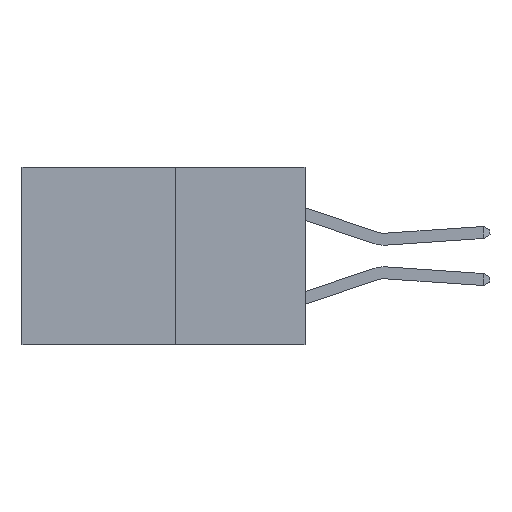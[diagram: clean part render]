
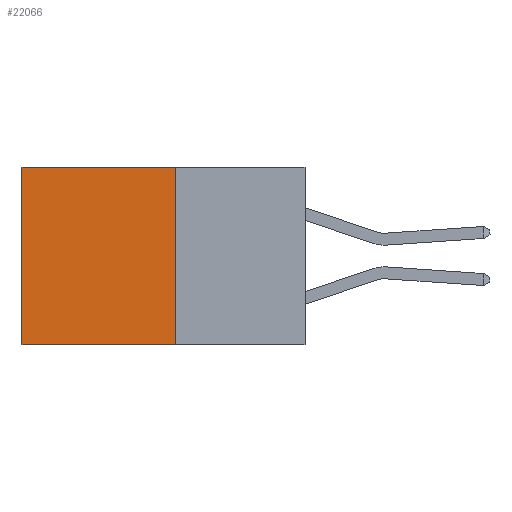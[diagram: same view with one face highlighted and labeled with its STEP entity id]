
A CAD part, left-side view. The second image highlights one B-rep face of the part: STEP entity #22066.
In plain terms, the highlighted planar face has unit normal (-1, 0, 0).
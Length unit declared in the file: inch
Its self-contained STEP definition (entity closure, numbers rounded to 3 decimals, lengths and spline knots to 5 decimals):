
#413 = ORIENTED_EDGE ( 'NONE', *, *, #15165, .F. ) ;
#3929 = CARTESIAN_POINT ( 'NONE',  ( 0.277, 0.27, 0. ) ) ;
#4250 = DIRECTION ( 'NONE',  ( 0., 0., -1. ) ) ;
#4653 = LINE ( 'NONE', #3929, #33770 ) ;
#5670 = VECTOR ( 'NONE', #6092, 39.37008 ) ;
#6092 = DIRECTION ( 'NONE',  ( 0., 0., -1. ) ) ;
#6223 = CARTESIAN_POINT ( 'NONE',  ( 0.277, 0.59, 0. ) ) ;
#6736 = ORIENTED_EDGE ( 'NONE', *, *, #20087, .T. ) ;
#7680 = ORIENTED_EDGE ( 'NONE', *, *, #29803, .T. ) ;
#7690 = VECTOR ( 'NONE', #10280, 39.37008 ) ;
#8318 = EDGE_LOOP ( 'NONE', ( #6736, #413, #28254, #7680 ) ) ;
#9509 = CARTESIAN_POINT ( 'NONE',  ( 0.277, 0.27, -0.37 ) ) ;
#10280 = DIRECTION ( 'NONE',  ( 0., 1., 0. ) ) ;
#10486 = CARTESIAN_POINT ( 'NONE',  ( 0.277, 0.27, -0.37 ) ) ;
#11647 = VERTEX_POINT ( 'NONE', #32104 ) ;
#12366 = PLANE ( 'NONE',  #14031 ) ;
#13124 = CARTESIAN_POINT ( 'NONE',  ( 0.277, 0.27, -0.37 ) ) ;
#14031 = AXIS2_PLACEMENT_3D ( 'NONE', #9509, #15206, #34837 ) ;
#15165 = EDGE_CURVE ( 'NONE', #30581, #22522, #22787, .T. ) ;
#15206 = DIRECTION ( 'NONE',  ( 1., 0., 0. ) ) ;
#20087 = EDGE_CURVE ( 'NONE', #32452, #22522, #35589, .T. ) ;
#21642 = LINE ( 'NONE', #28567, #5670 ) ;
#22066 = ADVANCED_FACE ( 'NONE', ( #31579 ), #12366, .F. ) ;
#22522 = VERTEX_POINT ( 'NONE', #33965 ) ;
#22787 = LINE ( 'NONE', #13124, #7690 ) ;
#26542 = DIRECTION ( 'NONE',  ( 0., 1., 0. ) ) ;
#27290 = VECTOR ( 'NONE', #4250, 39.37008 ) ;
#28254 = ORIENTED_EDGE ( 'NONE', *, *, #34687, .F. ) ;
#28567 = CARTESIAN_POINT ( 'NONE',  ( 0.277, 0.27, -0.37 ) ) ;
#29573 = CARTESIAN_POINT ( 'NONE',  ( 0.277, 0.59, -0.37 ) ) ;
#29803 = EDGE_CURVE ( 'NONE', #11647, #32452, #4653, .T. ) ;
#30581 = VERTEX_POINT ( 'NONE', #10486 ) ;
#31579 = FACE_OUTER_BOUND ( 'NONE', #8318, .T. ) ;
#32104 = CARTESIAN_POINT ( 'NONE',  ( 0.277, 0.27, 0. ) ) ;
#32452 = VERTEX_POINT ( 'NONE', #6223 ) ;
#33770 = VECTOR ( 'NONE', #26542, 39.37008 ) ;
#33965 = CARTESIAN_POINT ( 'NONE',  ( 0.277, 0.59, -0.37 ) ) ;
#34687 = EDGE_CURVE ( 'NONE', #11647, #30581, #21642, .T. ) ;
#34837 = DIRECTION ( 'NONE',  ( 0., 0., -1. ) ) ;
#35589 = LINE ( 'NONE', #29573, #27290 ) ;
